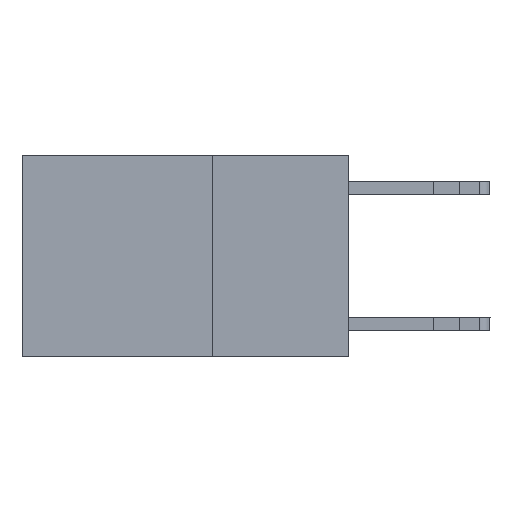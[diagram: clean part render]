
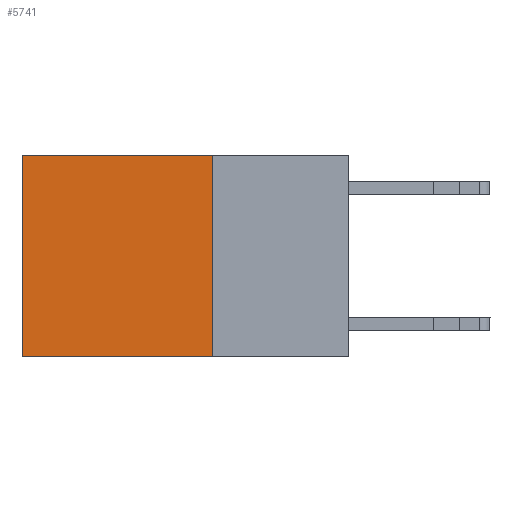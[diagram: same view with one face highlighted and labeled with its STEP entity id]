
A CAD part, left-side view. The second image highlights one B-rep face of the part: STEP entity #5741.
In plain terms, the highlighted planar face has unit normal (-1, 0, 0).
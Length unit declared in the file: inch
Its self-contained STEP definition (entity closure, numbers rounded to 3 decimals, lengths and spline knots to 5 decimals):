
#104 = DIRECTION ( 'NONE',  ( 1., 0., 0. ) ) ;
#153 = PLANE ( 'NONE',  #23901 ) ;
#1178 = CARTESIAN_POINT ( 'NONE',  ( 0.2625, 0.25, 0. ) ) ;
#1257 = EDGE_CURVE ( 'NONE', #16009, #24944, #14413, .T. ) ;
#2064 = CARTESIAN_POINT ( 'NONE',  ( 0.2625, 0.25, -0.37 ) ) ;
#2377 = DIRECTION ( 'NONE',  ( 0., 1., 0. ) ) ;
#2779 = ORIENTED_EDGE ( 'NONE', *, *, #6057, .T. ) ;
#3064 = VERTEX_POINT ( 'NONE', #23936 ) ;
#5741 = ADVANCED_FACE ( 'NONE', ( #12581 ), #153, .F. ) ;
#6057 = EDGE_CURVE ( 'NONE', #3064, #21649, #8734, .T. ) ;
#8734 = LINE ( 'NONE', #16651, #8861 ) ;
#8861 = VECTOR ( 'NONE', #16626, 39.37008 ) ;
#9895 = DIRECTION ( 'NONE',  ( 0., 1., 0. ) ) ;
#9980 = CARTESIAN_POINT ( 'NONE',  ( 0.2625, 0.25, 0. ) ) ;
#10209 = EDGE_CURVE ( 'NONE', #16009, #3064, #20250, .T. ) ;
#11967 = ORIENTED_EDGE ( 'NONE', *, *, #1257, .F. ) ;
#12190 = EDGE_LOOP ( 'NONE', ( #2779, #15058, #11967, #17876 ) ) ;
#12581 = FACE_OUTER_BOUND ( 'NONE', #12190, .T. ) ;
#12929 = EDGE_CURVE ( 'NONE', #24944, #21649, #24767, .T. ) ;
#14413 = LINE ( 'NONE', #21833, #14504 ) ;
#14504 = VECTOR ( 'NONE', #21812, 39.37008 ) ;
#15058 = ORIENTED_EDGE ( 'NONE', *, *, #12929, .F. ) ;
#16009 = VERTEX_POINT ( 'NONE', #18907 ) ;
#16495 = CARTESIAN_POINT ( 'NONE',  ( 0.2625, 0.25, -0.37 ) ) ;
#16626 = DIRECTION ( 'NONE',  ( 0., 0., -1. ) ) ;
#16651 = CARTESIAN_POINT ( 'NONE',  ( 0.2625, 0.6, 0. ) ) ;
#17876 = ORIENTED_EDGE ( 'NONE', *, *, #10209, .T. ) ;
#17953 = CARTESIAN_POINT ( 'NONE',  ( 0.2625, 0.6, -0.37 ) ) ;
#18907 = CARTESIAN_POINT ( 'NONE',  ( 0.2625, 0.25, 0. ) ) ;
#19923 = VECTOR ( 'NONE', #9895, 39.37008 ) ;
#20250 = LINE ( 'NONE', #9980, #19923 ) ;
#21649 = VERTEX_POINT ( 'NONE', #17953 ) ;
#21812 = DIRECTION ( 'NONE',  ( 0., 0., -1. ) ) ;
#21833 = CARTESIAN_POINT ( 'NONE',  ( 0.2625, 0.25, 0. ) ) ;
#23901 = AXIS2_PLACEMENT_3D ( 'NONE', #1178, #104, #25204 ) ;
#23936 = CARTESIAN_POINT ( 'NONE',  ( 0.2625, 0.6, 0. ) ) ;
#24686 = VECTOR ( 'NONE', #2377, 39.37008 ) ;
#24767 = LINE ( 'NONE', #2064, #24686 ) ;
#24944 = VERTEX_POINT ( 'NONE', #16495 ) ;
#25204 = DIRECTION ( 'NONE',  ( 0., 0., -1. ) ) ;
